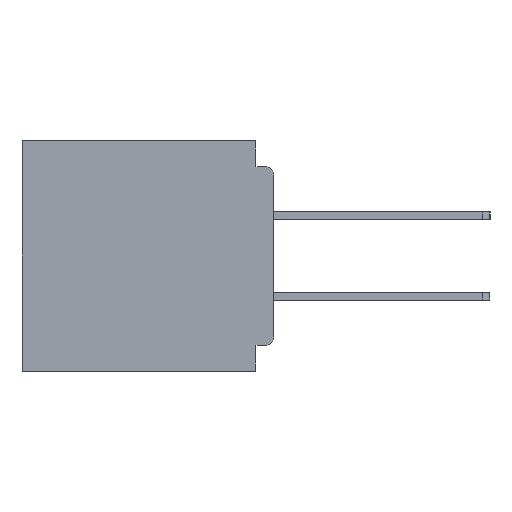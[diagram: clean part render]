
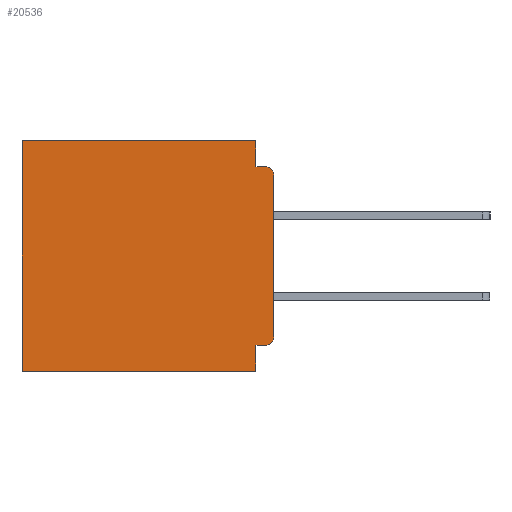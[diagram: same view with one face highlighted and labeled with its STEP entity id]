
A CAD part, left-side view. The second image highlights one B-rep face of the part: STEP entity #20536.
In plain terms, the highlighted planar face has unit normal (-1, 0, 0).
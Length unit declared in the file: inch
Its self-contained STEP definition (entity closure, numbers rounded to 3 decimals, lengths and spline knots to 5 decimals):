
#897 = CARTESIAN_POINT ( 'NONE',  ( 0.3, 0.031, -0.355 ) ) ;
#963 = CARTESIAN_POINT ( 'NONE',  ( 0.3, 0.015, -0.045 ) ) ;
#971 = CARTESIAN_POINT ( 'NONE',  ( 0.3, 0.015, -0.06 ) ) ;
#1662 = CIRCLE ( 'NONE', #35997, 0.015 ) ;
#1890 = EDGE_CURVE ( 'NONE', #36588, #37063, #5343, .T. ) ;
#3172 = CARTESIAN_POINT ( 'NONE',  ( 0.3, 0., -0.4 ) ) ;
#3377 = DIRECTION ( 'NONE',  ( 0., 0., -1. ) ) ;
#4051 = DIRECTION ( 'NONE',  ( 0., 0., -1. ) ) ;
#4404 = VECTOR ( 'NONE', #3377, 39.37008 ) ;
#4797 = LINE ( 'NONE', #25677, #25413 ) ;
#5201 = CARTESIAN_POINT ( 'NONE',  ( 0.3, 0.437, -0.4 ) ) ;
#5343 = LINE ( 'NONE', #3172, #4404 ) ;
#6034 = ORIENTED_EDGE ( 'NONE', *, *, #12055, .T. ) ;
#6068 = VERTEX_POINT ( 'NONE', #963 ) ;
#7050 = VECTOR ( 'NONE', #25545, 39.37008 ) ;
#7966 = LINE ( 'NONE', #5201, #7050 ) ;
#8126 = CARTESIAN_POINT ( 'NONE',  ( 0.3, 0.437, -0.4 ) ) ;
#8472 = DIRECTION ( 'NONE',  ( 0., 1., 0. ) ) ;
#8529 = EDGE_CURVE ( 'NONE', #11274, #26526, #36872, .T. ) ;
#8832 = CARTESIAN_POINT ( 'NONE',  ( 0.3, 0.031, -0.4 ) ) ;
#8860 = DIRECTION ( 'NONE',  ( 0., 0., -1. ) ) ;
#9055 = ORIENTED_EDGE ( 'NONE', *, *, #26281, .T. ) ;
#9683 = VERTEX_POINT ( 'NONE', #8126 ) ;
#9963 = ORIENTED_EDGE ( 'NONE', *, *, #22468, .F. ) ;
#10140 = ORIENTED_EDGE ( 'NONE', *, *, #1890, .F. ) ;
#10204 = VECTOR ( 'NONE', #15702, 39.37008 ) ;
#10351 = PLANE ( 'NONE',  #32690 ) ;
#10547 = EDGE_CURVE ( 'NONE', #11274, #20738, #29767, .T. ) ;
#10584 = ORIENTED_EDGE ( 'NONE', *, *, #20411, .F. ) ;
#10645 = CARTESIAN_POINT ( 'NONE',  ( 0.3, 0., -0.06 ) ) ;
#11002 = ORIENTED_EDGE ( 'NONE', *, *, #30561, .F. ) ;
#11274 = VERTEX_POINT ( 'NONE', #35221 ) ;
#11386 = VERTEX_POINT ( 'NONE', #897 ) ;
#11459 = CARTESIAN_POINT ( 'NONE',  ( 0.3, 0., -0.355 ) ) ;
#11666 = ORIENTED_EDGE ( 'NONE', *, *, #10547, .T. ) ;
#12055 = EDGE_CURVE ( 'NONE', #36588, #6068, #1662, .T. ) ;
#12070 = ORIENTED_EDGE ( 'NONE', *, *, #25472, .T. ) ;
#12274 = ORIENTED_EDGE ( 'NONE', *, *, #8529, .F. ) ;
#13326 = DIRECTION ( 'NONE',  ( 0., 0., -1. ) ) ;
#14202 = ORIENTED_EDGE ( 'NONE', *, *, #32857, .F. ) ;
#15702 = DIRECTION ( 'NONE',  ( 0., 0., -1. ) ) ;
#16961 = DIRECTION ( 'NONE',  ( 0., -1., 0. ) ) ;
#17657 = DIRECTION ( 'NONE',  ( -1., 0., 0. ) ) ;
#18078 = LINE ( 'NONE', #30001, #10204 ) ;
#19614 = EDGE_LOOP ( 'NONE', ( #10140, #6034, #9963, #12274, #11666, #12070, #11002, #10584, #14202, #9055 ) ) ;
#20037 = CARTESIAN_POINT ( 'NONE',  ( 0.3, 0.015, -0.355 ) ) ;
#20411 = EDGE_CURVE ( 'NONE', #11386, #33418, #18078, .T. ) ;
#20536 = ADVANCED_FACE ( 'NONE', ( #35358 ), #10351, .F. ) ;
#20738 = VERTEX_POINT ( 'NONE', #22879 ) ;
#21584 = CARTESIAN_POINT ( 'NONE',  ( 0.3, 0., 0. ) ) ;
#21729 = DIRECTION ( 'NONE',  ( -1., 0., 0. ) ) ;
#22226 = VECTOR ( 'NONE', #8472, 39.37008 ) ;
#22468 = EDGE_CURVE ( 'NONE', #26526, #6068, #31354, .T. ) ;
#22879 = CARTESIAN_POINT ( 'NONE',  ( 0.3, 0.437, 0. ) ) ;
#24362 = CIRCLE ( 'NONE', #32137, 0.015 ) ;
#25014 = CARTESIAN_POINT ( 'NONE',  ( 0.3, 0., -0.34 ) ) ;
#25413 = VECTOR ( 'NONE', #34179, 39.37008 ) ;
#25472 = EDGE_CURVE ( 'NONE', #20738, #9683, #7966, .T. ) ;
#25545 = DIRECTION ( 'NONE',  ( 0., 0., -1. ) ) ;
#25677 = CARTESIAN_POINT ( 'NONE',  ( 0.3, 0., -0.4 ) ) ;
#26281 = EDGE_CURVE ( 'NONE', #34355, #37063, #24362, .T. ) ;
#26297 = CARTESIAN_POINT ( 'NONE',  ( 0.3, 0.031, 0. ) ) ;
#26526 = VERTEX_POINT ( 'NONE', #35735 ) ;
#27294 = DIRECTION ( 'NONE',  ( 0., 1., 0. ) ) ;
#27723 = CARTESIAN_POINT ( 'NONE',  ( 0.3, 0., -0.4 ) ) ;
#29447 = VECTOR ( 'NONE', #8860, 39.37008 ) ;
#29767 = LINE ( 'NONE', #21584, #36283 ) ;
#30001 = CARTESIAN_POINT ( 'NONE',  ( 0.3, 0.031, -0.4 ) ) ;
#30471 = VECTOR ( 'NONE', #16961, 39.37008 ) ;
#30561 = EDGE_CURVE ( 'NONE', #33418, #9683, #4797, .T. ) ;
#30589 = DIRECTION ( 'NONE',  ( 1., 0., 0. ) ) ;
#31215 = CARTESIAN_POINT ( 'NONE',  ( 0.3, 0., -0.045 ) ) ;
#31354 = LINE ( 'NONE', #31215, #30471 ) ;
#32137 = AXIS2_PLACEMENT_3D ( 'NONE', #34663, #17657, #37456 ) ;
#32690 = AXIS2_PLACEMENT_3D ( 'NONE', #27723, #30589, #13326 ) ;
#32857 = EDGE_CURVE ( 'NONE', #34355, #11386, #37186, .T. ) ;
#33418 = VERTEX_POINT ( 'NONE', #8832 ) ;
#34179 = DIRECTION ( 'NONE',  ( 0., 1., 0. ) ) ;
#34355 = VERTEX_POINT ( 'NONE', #20037 ) ;
#34663 = CARTESIAN_POINT ( 'NONE',  ( 0.3, 0.015, -0.34 ) ) ;
#35221 = CARTESIAN_POINT ( 'NONE',  ( 0.3, 0.031, 0. ) ) ;
#35358 = FACE_OUTER_BOUND ( 'NONE', #19614, .T. ) ;
#35735 = CARTESIAN_POINT ( 'NONE',  ( 0.3, 0.031, -0.045 ) ) ;
#35997 = AXIS2_PLACEMENT_3D ( 'NONE', #971, #21729, #4051 ) ;
#36283 = VECTOR ( 'NONE', #27294, 39.37008 ) ;
#36588 = VERTEX_POINT ( 'NONE', #10645 ) ;
#36872 = LINE ( 'NONE', #26297, #29447 ) ;
#37063 = VERTEX_POINT ( 'NONE', #25014 ) ;
#37186 = LINE ( 'NONE', #11459, #22226 ) ;
#37456 = DIRECTION ( 'NONE',  ( 0., 0., -1. ) ) ;
